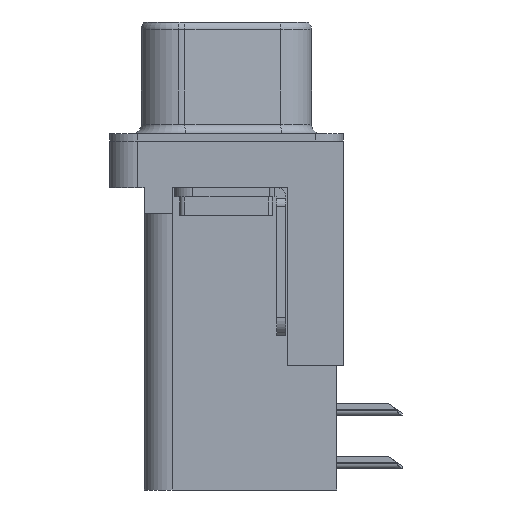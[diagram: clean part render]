
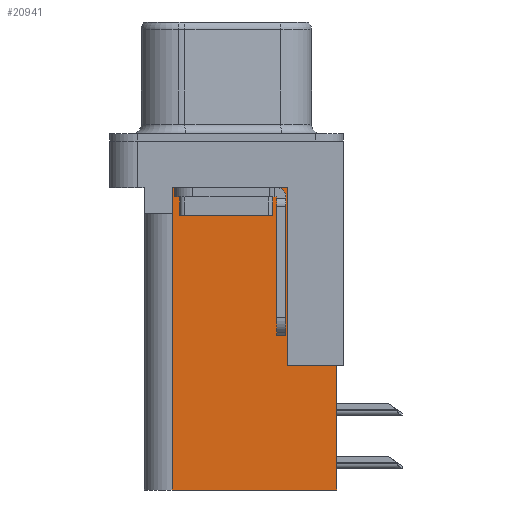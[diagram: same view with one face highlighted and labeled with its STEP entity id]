
A CAD part, left-side view. The second image highlights one B-rep face of the part: STEP entity #20941.
In plain terms, the highlighted planar face has unit normal (-1, 0, 0).
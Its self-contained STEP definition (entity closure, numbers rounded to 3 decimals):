
#327 = DIRECTION ( 'NONE',  ( 0., 0., 1. ) ) ;
#676 = DIRECTION ( 'NONE',  ( 0., 1., 0. ) ) ;
#790 = VECTOR ( 'NONE', #11673, 1000. ) ;
#1237 = VERTEX_POINT ( 'NONE', #1470 ) ;
#1470 = CARTESIAN_POINT ( 'NONE',  ( 3.79, 2.895, -3.9 ) ) ;
#2321 = CARTESIAN_POINT ( 'NONE',  ( 3.79, -6.295, -12.05 ) ) ;
#2482 = VERTEX_POINT ( 'NONE', #12407 ) ;
#2817 = CARTESIAN_POINT ( 'NONE',  ( 3.79, -3.295, -2.5 ) ) ;
#3921 = DIRECTION ( 'NONE',  ( 0., 1., 0. ) ) ;
#3973 = AXIS2_PLACEMENT_3D ( 'NONE', #10261, #24665, #12357 ) ;
#4083 = CARTESIAN_POINT ( 'NONE',  ( 3.79, 2.925, -18.76 ) ) ;
#4226 = ORIENTED_EDGE ( 'NONE', *, *, #8183, .T. ) ;
#4422 = VECTOR ( 'NONE', #24582, 1000. ) ;
#4473 = VERTEX_POINT ( 'NONE', #25033 ) ;
#4592 = CARTESIAN_POINT ( 'NONE',  ( 3.79, -5.925, -18.76 ) ) ;
#5612 = EDGE_CURVE ( 'NONE', #2482, #1237, #8264, .T. ) ;
#5779 = CARTESIAN_POINT ( 'NONE',  ( 3.79, -5.925, -12.05 ) ) ;
#5788 = ORIENTED_EDGE ( 'NONE', *, *, #8064, .F. ) ;
#6246 = LINE ( 'NONE', #4083, #790 ) ;
#6656 = LINE ( 'NONE', #2321, #22408 ) ;
#6940 = EDGE_CURVE ( 'NONE', #1237, #13935, #24271, .T. ) ;
#7331 = EDGE_CURVE ( 'NONE', #4473, #13935, #6246, .T. ) ;
#7939 = CARTESIAN_POINT ( 'NONE',  ( 3.79, 0., -3.9 ) ) ;
#7991 = EDGE_CURVE ( 'NONE', #19379, #4473, #26270, .T. ) ;
#8064 = EDGE_CURVE ( 'NONE', #19142, #19379, #19568, .T. ) ;
#8148 = EDGE_CURVE ( 'NONE', #19142, #9322, #6656, .T. ) ;
#8183 = EDGE_CURVE ( 'NONE', #9322, #12267, #23033, .T. ) ;
#8264 = LINE ( 'NONE', #13073, #13724 ) ;
#8508 = CARTESIAN_POINT ( 'NONE',  ( 3.79, -3.295, -18.76 ) ) ;
#9322 = VERTEX_POINT ( 'NONE', #16716 ) ;
#9873 = VECTOR ( 'NONE', #3921, 1000. ) ;
#10028 = DIRECTION ( 'NONE',  ( 0., 1., 0. ) ) ;
#10261 = CARTESIAN_POINT ( 'NONE',  ( 3.79, -3.295, -18.76 ) ) ;
#10580 = ORIENTED_EDGE ( 'NONE', *, *, #8148, .T. ) ;
#10684 = VECTOR ( 'NONE', #10028, 1000. ) ;
#10813 = ORIENTED_EDGE ( 'NONE', *, *, #6940, .T. ) ;
#11334 = EDGE_CURVE ( 'NONE', #12267, #2482, #16199, .T. ) ;
#11673 = DIRECTION ( 'NONE',  ( 0., 0., 1. ) ) ;
#11985 = DIRECTION ( 'NONE',  ( 0., 0., -1. ) ) ;
#12267 = VERTEX_POINT ( 'NONE', #2817 ) ;
#12272 = CARTESIAN_POINT ( 'NONE',  ( 3.79, -5.925, -2. ) ) ;
#12357 = DIRECTION ( 'NONE',  ( 0., 1., 0. ) ) ;
#12407 = CARTESIAN_POINT ( 'NONE',  ( 3.79, 2.895, -2.5 ) ) ;
#12605 = CARTESIAN_POINT ( 'NONE',  ( 3.79, 2.925, -3.9 ) ) ;
#13073 = CARTESIAN_POINT ( 'NONE',  ( 3.79, 2.895, -3.9 ) ) ;
#13724 = VECTOR ( 'NONE', #11985, 1000. ) ;
#13935 = VERTEX_POINT ( 'NONE', #12605 ) ;
#14637 = DIRECTION ( 'NONE',  ( 0., 1., 0. ) ) ;
#14977 = ORIENTED_EDGE ( 'NONE', *, *, #5612, .T. ) ;
#16199 = LINE ( 'NONE', #22339, #10684 ) ;
#16245 = EDGE_LOOP ( 'NONE', ( #24600, #14977, #10813, #19695, #22220, #5788, #10580, #4226 ) ) ;
#16330 = VECTOR ( 'NONE', #327, 1000. ) ;
#16716 = CARTESIAN_POINT ( 'NONE',  ( 3.79, -3.295, -12.05 ) ) ;
#18858 = VECTOR ( 'NONE', #676, 1000. ) ;
#19142 = VERTEX_POINT ( 'NONE', #5779 ) ;
#19379 = VERTEX_POINT ( 'NONE', #4592 ) ;
#19568 = LINE ( 'NONE', #12272, #4422 ) ;
#19695 = ORIENTED_EDGE ( 'NONE', *, *, #7331, .F. ) ;
#20941 = ADVANCED_FACE ( 'NONE', ( #21039 ), #24384, .F. ) ;
#21039 = FACE_OUTER_BOUND ( 'NONE', #16245, .T. ) ;
#22220 = ORIENTED_EDGE ( 'NONE', *, *, #7991, .F. ) ;
#22339 = CARTESIAN_POINT ( 'NONE',  ( 3.79, -3.295, -2.5 ) ) ;
#22408 = VECTOR ( 'NONE', #14637, 1000. ) ;
#23033 = LINE ( 'NONE', #8508, #16330 ) ;
#24271 = LINE ( 'NONE', #7939, #18858 ) ;
#24384 = PLANE ( 'NONE',  #3973 ) ;
#24582 = DIRECTION ( 'NONE',  ( 0., 0., -1. ) ) ;
#24600 = ORIENTED_EDGE ( 'NONE', *, *, #11334, .T. ) ;
#24665 = DIRECTION ( 'NONE',  ( 1., 0., 0. ) ) ;
#25033 = CARTESIAN_POINT ( 'NONE',  ( 3.79, 2.925, -18.76 ) ) ;
#26270 = LINE ( 'NONE', #26375, #9873 ) ;
#26375 = CARTESIAN_POINT ( 'NONE',  ( 3.79, -3.295, -18.76 ) ) ;
